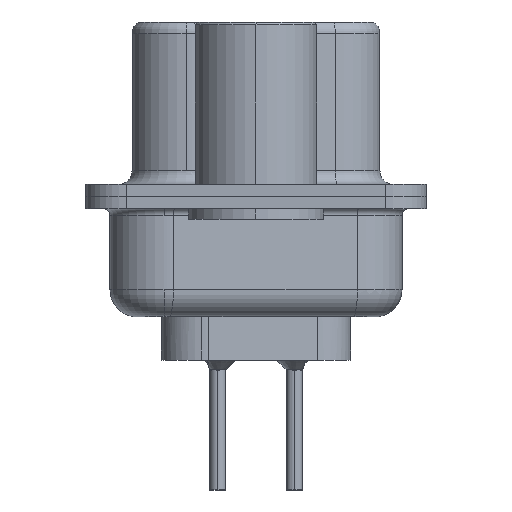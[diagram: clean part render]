
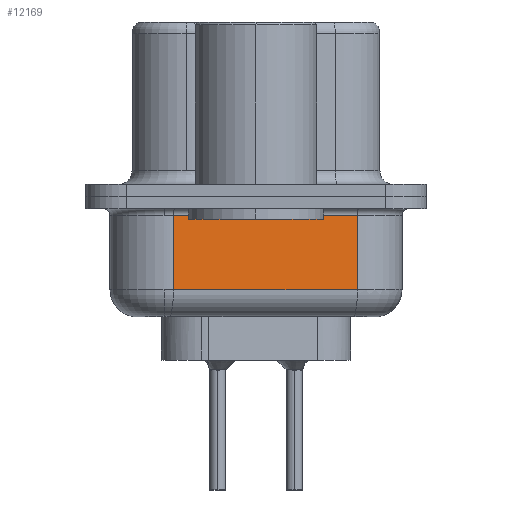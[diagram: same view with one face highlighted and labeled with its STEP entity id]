
A CAD part, left-side view. The second image highlights one B-rep face of the part: STEP entity #12169.
In plain terms, the highlighted planar face has unit normal (-0.985, -0.174, 0).
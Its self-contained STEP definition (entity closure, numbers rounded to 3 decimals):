
#590 = VERTEX_POINT ( 'NONE', #2809 ) ;
#967 = CARTESIAN_POINT ( 'NONE',  ( 2.85, 3.053, -0.7 ) ) ;
#1517 = CARTESIAN_POINT ( 'NONE',  ( 4.049, -3.747, -4.45 ) ) ;
#2809 = CARTESIAN_POINT ( 'NONE',  ( 2.85, 3.053, -3.45 ) ) ;
#3553 = PLANE ( 'NONE',  #21649 ) ;
#4198 = VERTEX_POINT ( 'NONE', #18029 ) ;
#4379 = LINE ( 'NONE', #14628, #4744 ) ;
#4744 = VECTOR ( 'NONE', #12786, 1000. ) ;
#5000 = LINE ( 'NONE', #6848, #7284 ) ;
#5257 = ORIENTED_EDGE ( 'NONE', *, *, #7515, .F. ) ;
#5825 = ORIENTED_EDGE ( 'NONE', *, *, #21001, .T. ) ;
#5980 = ORIENTED_EDGE ( 'NONE', *, *, #14414, .T. ) ;
#6719 = DIRECTION ( 'NONE',  ( 0., 0., 1. ) ) ;
#6848 = CARTESIAN_POINT ( 'NONE',  ( 2.85, 3.053, -4.45 ) ) ;
#7184 = LINE ( 'NONE', #1517, #11646 ) ;
#7284 = VECTOR ( 'NONE', #6719, 1000. ) ;
#7515 = EDGE_CURVE ( 'NONE', #590, #19679, #5000, .T. ) ;
#7603 = DIRECTION ( 'NONE',  ( -0.174, 0.985, 0. ) ) ;
#9703 = ORIENTED_EDGE ( 'NONE', *, *, #22253, .T. ) ;
#11362 = DIRECTION ( 'NONE',  ( 0., 0., 1. ) ) ;
#11646 = VECTOR ( 'NONE', #11362, 1000. ) ;
#12169 = ADVANCED_FACE ( 'NONE', ( #15086 ), #3553, .F. ) ;
#12175 = EDGE_LOOP ( 'NONE', ( #5257, #5825, #5980, #9703 ) ) ;
#12786 = DIRECTION ( 'NONE',  ( 0.174, -0.985, 0. ) ) ;
#13885 = CARTESIAN_POINT ( 'NONE',  ( 2.85, 3.053, -0.7 ) ) ;
#14389 = VERTEX_POINT ( 'NONE', #21191 ) ;
#14414 = EDGE_CURVE ( 'NONE', #14389, #4198, #7184, .T. ) ;
#14628 = CARTESIAN_POINT ( 'NONE',  ( 2.85, 3.053, -3.45 ) ) ;
#15086 = FACE_OUTER_BOUND ( 'NONE', #12175, .T. ) ;
#17187 = DIRECTION ( 'NONE',  ( -0.174, 0.985, 0. ) ) ;
#18029 = CARTESIAN_POINT ( 'NONE',  ( 4.049, -3.747, -0.7 ) ) ;
#19304 = CARTESIAN_POINT ( 'NONE',  ( 2.85, 3.053, -4.45 ) ) ;
#19679 = VERTEX_POINT ( 'NONE', #967 ) ;
#21001 = EDGE_CURVE ( 'NONE', #590, #14389, #4379, .T. ) ;
#21191 = CARTESIAN_POINT ( 'NONE',  ( 4.049, -3.747, -3.45 ) ) ;
#21624 = LINE ( 'NONE', #13885, #24500 ) ;
#21649 = AXIS2_PLACEMENT_3D ( 'NONE', #19304, #25573, #17187 ) ;
#22253 = EDGE_CURVE ( 'NONE', #4198, #19679, #21624, .T. ) ;
#24500 = VECTOR ( 'NONE', #7603, 1000. ) ;
#25573 = DIRECTION ( 'NONE',  ( 0.985, 0.174, 0. ) ) ;
